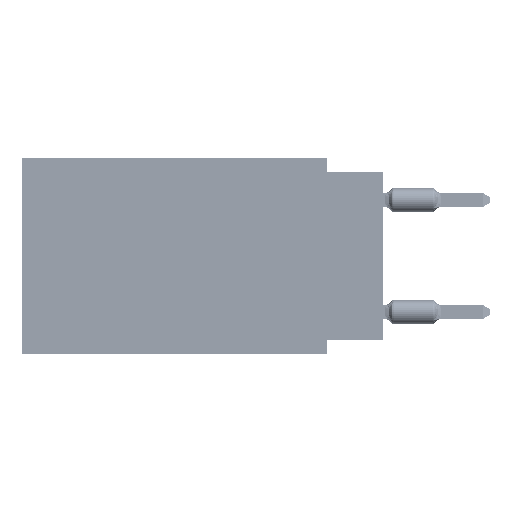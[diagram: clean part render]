
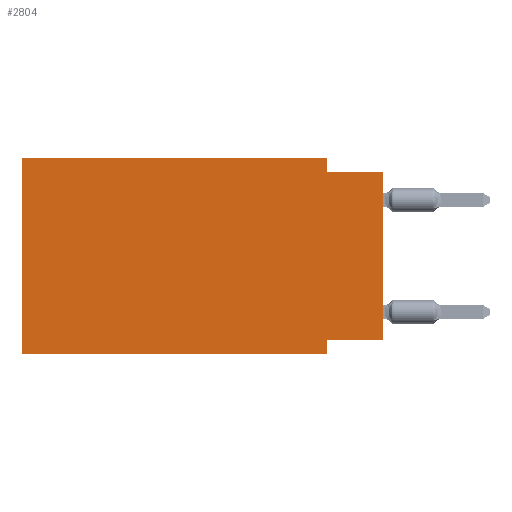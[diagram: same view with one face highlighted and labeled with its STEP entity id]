
A CAD part, left-side view. The second image highlights one B-rep face of the part: STEP entity #2804.
In plain terms, the highlighted planar face has unit normal (-1, 0, 0).
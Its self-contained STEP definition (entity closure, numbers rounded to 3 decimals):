
#150 = EDGE_CURVE ( 'NONE', #42354, #10428, #13981, .T. ) ;
#1354 = CARTESIAN_POINT ( 'NONE',  ( 0., 0., -0.635 ) ) ;
#2804 = ADVANCED_FACE ( 'NONE', ( #61834 ), #91868, .F. ) ;
#4315 = VERTEX_POINT ( 'NONE', #85494 ) ;
#5146 = LINE ( 'NONE', #27825, #59113 ) ;
#6355 = ORIENTED_EDGE ( 'NONE', *, *, #78101, .F. ) ;
#7689 = DIRECTION ( 'NONE',  ( 1., 0., 0. ) ) ;
#10428 = VERTEX_POINT ( 'NONE', #55014 ) ;
#13981 = LINE ( 'NONE', #59263, #74754 ) ;
#15443 = VERTEX_POINT ( 'NONE', #36543 ) ;
#17028 = DIRECTION ( 'NONE',  ( 0., -1., 0. ) ) ;
#17132 = LINE ( 'NONE', #1354, #46253 ) ;
#18118 = VERTEX_POINT ( 'NONE', #96567 ) ;
#20149 = AXIS2_PLACEMENT_3D ( 'NONE', #39680, #7689, #83035 ) ;
#22277 = ORIENTED_EDGE ( 'NONE', *, *, #24357, .F. ) ;
#22363 = CARTESIAN_POINT ( 'NONE',  ( 0., 16.383, -8.89 ) ) ;
#22550 = VECTOR ( 'NONE', #87565, 1000. ) ;
#24357 = EDGE_CURVE ( 'NONE', #4315, #73862, #50618, .T. ) ;
#27825 = CARTESIAN_POINT ( 'NONE',  ( 0., 16.383, 0. ) ) ;
#30851 = ORIENTED_EDGE ( 'NONE', *, *, #47269, .F. ) ;
#31390 = EDGE_CURVE ( 'NONE', #95965, #4315, #35465, .T. ) ;
#33749 = DIRECTION ( 'NONE',  ( 0., -1., 0. ) ) ;
#35465 = LINE ( 'NONE', #95497, #61679 ) ;
#35757 = EDGE_CURVE ( 'NONE', #42354, #73862, #55913, .T. ) ;
#36543 = CARTESIAN_POINT ( 'NONE',  ( 0., 2.54, 0. ) ) ;
#37268 = VECTOR ( 'NONE', #37338, 1000. ) ;
#37338 = DIRECTION ( 'NONE',  ( 0., 0., 1. ) ) ;
#37626 = EDGE_LOOP ( 'NONE', ( #72407, #71985, #6355, #30851, #82215, #63451, #22277, #90919 ) ) ;
#39680 = CARTESIAN_POINT ( 'NONE',  ( 0., 16.383, 0. ) ) ;
#40152 = CARTESIAN_POINT ( 'NONE',  ( 0., 16.383, -8.89 ) ) ;
#42354 = VERTEX_POINT ( 'NONE', #22363 ) ;
#45390 = EDGE_CURVE ( 'NONE', #45839, #18118, #17132, .T. ) ;
#45839 = VERTEX_POINT ( 'NONE', #77567 ) ;
#46253 = VECTOR ( 'NONE', #47143, 1000. ) ;
#47143 = DIRECTION ( 'NONE',  ( 0., -1., 0. ) ) ;
#47269 = EDGE_CURVE ( 'NONE', #10428, #15443, #5146, .T. ) ;
#47734 = CARTESIAN_POINT ( 'NONE',  ( 0., 0., -8.255 ) ) ;
#47958 = EDGE_CURVE ( 'NONE', #95965, #18118, #74752, .T. ) ;
#50618 = LINE ( 'NONE', #59458, #22550 ) ;
#51277 = LINE ( 'NONE', #96537, #55786 ) ;
#52847 = DIRECTION ( 'NONE',  ( 0., 0., 1. ) ) ;
#55014 = CARTESIAN_POINT ( 'NONE',  ( 0., 16.383, 0. ) ) ;
#55786 = VECTOR ( 'NONE', #96055, 1000. ) ;
#55913 = LINE ( 'NONE', #40152, #73273 ) ;
#59113 = VECTOR ( 'NONE', #33749, 1000. ) ;
#59263 = CARTESIAN_POINT ( 'NONE',  ( 0., 16.383, 0. ) ) ;
#59458 = CARTESIAN_POINT ( 'NONE',  ( 0., 2.54, -8.89 ) ) ;
#59550 = CARTESIAN_POINT ( 'NONE',  ( 0., 2.54, -8.89 ) ) ;
#61679 = VECTOR ( 'NONE', #94049, 1000. ) ;
#61834 = FACE_OUTER_BOUND ( 'NONE', #37626, .T. ) ;
#63451 = ORIENTED_EDGE ( 'NONE', *, *, #35757, .T. ) ;
#71985 = ORIENTED_EDGE ( 'NONE', *, *, #45390, .F. ) ;
#72407 = ORIENTED_EDGE ( 'NONE', *, *, #47958, .T. ) ;
#73273 = VECTOR ( 'NONE', #17028, 1000. ) ;
#73862 = VERTEX_POINT ( 'NONE', #59550 ) ;
#74258 = CARTESIAN_POINT ( 'NONE',  ( 0., 0., 0. ) ) ;
#74752 = LINE ( 'NONE', #74258, #37268 ) ;
#74754 = VECTOR ( 'NONE', #52847, 1000. ) ;
#77567 = CARTESIAN_POINT ( 'NONE',  ( 0., 2.54, -0.635 ) ) ;
#78101 = EDGE_CURVE ( 'NONE', #15443, #45839, #51277, .T. ) ;
#82215 = ORIENTED_EDGE ( 'NONE', *, *, #150, .F. ) ;
#83035 = DIRECTION ( 'NONE',  ( 0., 0., -1. ) ) ;
#85494 = CARTESIAN_POINT ( 'NONE',  ( 0., 2.54, -8.255 ) ) ;
#87565 = DIRECTION ( 'NONE',  ( 0., 0., -1. ) ) ;
#90919 = ORIENTED_EDGE ( 'NONE', *, *, #31390, .F. ) ;
#91868 = PLANE ( 'NONE',  #20149 ) ;
#94049 = DIRECTION ( 'NONE',  ( 0., 1., 0. ) ) ;
#95497 = CARTESIAN_POINT ( 'NONE',  ( 0., 0., -8.255 ) ) ;
#95965 = VERTEX_POINT ( 'NONE', #47734 ) ;
#96055 = DIRECTION ( 'NONE',  ( 0., 0., -1. ) ) ;
#96537 = CARTESIAN_POINT ( 'NONE',  ( 0., 2.54, 0. ) ) ;
#96567 = CARTESIAN_POINT ( 'NONE',  ( 0., 0., -0.635 ) ) ;
